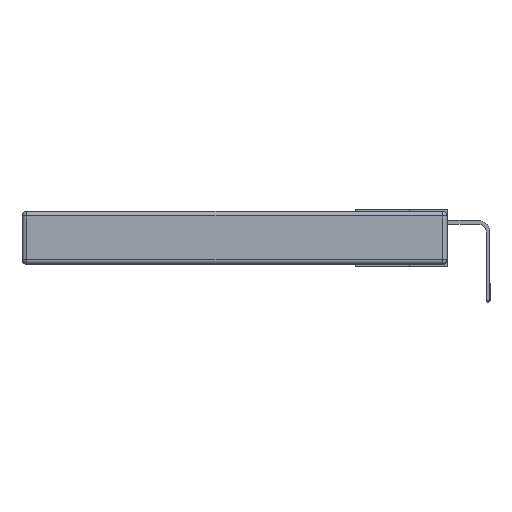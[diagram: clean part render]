
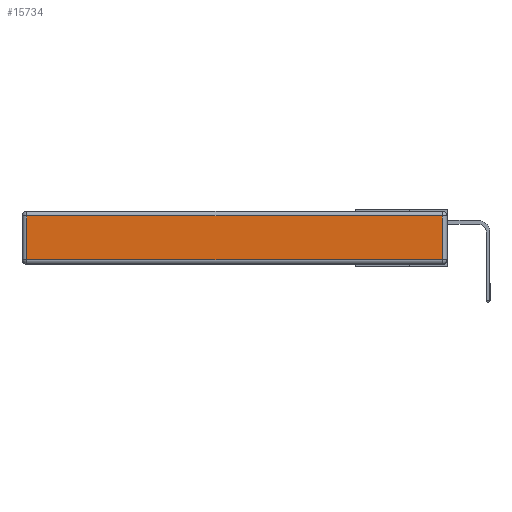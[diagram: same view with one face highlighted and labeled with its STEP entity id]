
A CAD part, left-side view. The second image highlights one B-rep face of the part: STEP entity #15734.
In plain terms, the highlighted planar face has unit normal (-1, 0, 0).
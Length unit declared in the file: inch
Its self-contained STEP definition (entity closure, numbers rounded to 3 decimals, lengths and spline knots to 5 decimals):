
#198 = VECTOR ( 'NONE', #26551, 39.37008 ) ;
#1039 = CARTESIAN_POINT ( 'NONE',  ( 0., 2.72, -0.313 ) ) ;
#1153 = CARTESIAN_POINT ( 'NONE',  ( 0., 0., -0.313 ) ) ;
#1702 = FACE_OUTER_BOUND ( 'NONE', #20555, .T. ) ;
#4399 = CARTESIAN_POINT ( 'NONE',  ( 0., 0.03, -0.313 ) ) ;
#4608 = PLANE ( 'NONE',  #9133 ) ;
#4864 = ORIENTED_EDGE ( 'NONE', *, *, #11835, .T. ) ;
#5401 = VECTOR ( 'NONE', #19981, 39.37008 ) ;
#7769 = VECTOR ( 'NONE', #24965, 39.37008 ) ;
#8546 = VECTOR ( 'NONE', #20527, 39.37008 ) ;
#8725 = VERTEX_POINT ( 'NONE', #1039 ) ;
#8945 = VERTEX_POINT ( 'NONE', #19893 ) ;
#9133 = AXIS2_PLACEMENT_3D ( 'NONE', #9355, #9268, #25383 ) ;
#9268 = DIRECTION ( 'NONE',  ( -1., 0., 0. ) ) ;
#9355 = CARTESIAN_POINT ( 'NONE',  ( 0., 0., -0.343 ) ) ;
#9550 = LINE ( 'NONE', #15406, #7769 ) ;
#9744 = VERTEX_POINT ( 'NONE', #4399 ) ;
#10490 = CARTESIAN_POINT ( 'NONE',  ( 0., 2.72, -0.03 ) ) ;
#11421 = LINE ( 'NONE', #13983, #8546 ) ;
#11835 = EDGE_CURVE ( 'NONE', #9744, #8945, #11421, .T. ) ;
#13983 = CARTESIAN_POINT ( 'NONE',  ( 0., 0.03, -0.343 ) ) ;
#14981 = ORIENTED_EDGE ( 'NONE', *, *, #22636, .T. ) ;
#15406 = CARTESIAN_POINT ( 'NONE',  ( 0., 2.75, -0.03 ) ) ;
#15734 = ADVANCED_FACE ( 'NONE', ( #1702 ), #4608, .T. ) ;
#16146 = EDGE_CURVE ( 'NONE', #8945, #18255, #9550, .T. ) ;
#16778 = EDGE_CURVE ( 'NONE', #18255, #8725, #27883, .T. ) ;
#18255 = VERTEX_POINT ( 'NONE', #10490 ) ;
#19625 = CARTESIAN_POINT ( 'NONE',  ( 0., 2.72, -0.343 ) ) ;
#19893 = CARTESIAN_POINT ( 'NONE',  ( 0., 0.03, -0.03 ) ) ;
#19981 = DIRECTION ( 'NONE',  ( 0., -1., 0. ) ) ;
#20527 = DIRECTION ( 'NONE',  ( 0., 0., 1. ) ) ;
#20555 = EDGE_LOOP ( 'NONE', ( #14981, #4864, #24585, #21159 ) ) ;
#21159 = ORIENTED_EDGE ( 'NONE', *, *, #16778, .T. ) ;
#22636 = EDGE_CURVE ( 'NONE', #8725, #9744, #27339, .T. ) ;
#24585 = ORIENTED_EDGE ( 'NONE', *, *, #16146, .T. ) ;
#24965 = DIRECTION ( 'NONE',  ( 0., 1., 0. ) ) ;
#25383 = DIRECTION ( 'NONE',  ( 0., 0., 1. ) ) ;
#26551 = DIRECTION ( 'NONE',  ( 0., 0., -1. ) ) ;
#27339 = LINE ( 'NONE', #1153, #5401 ) ;
#27883 = LINE ( 'NONE', #19625, #198 ) ;
